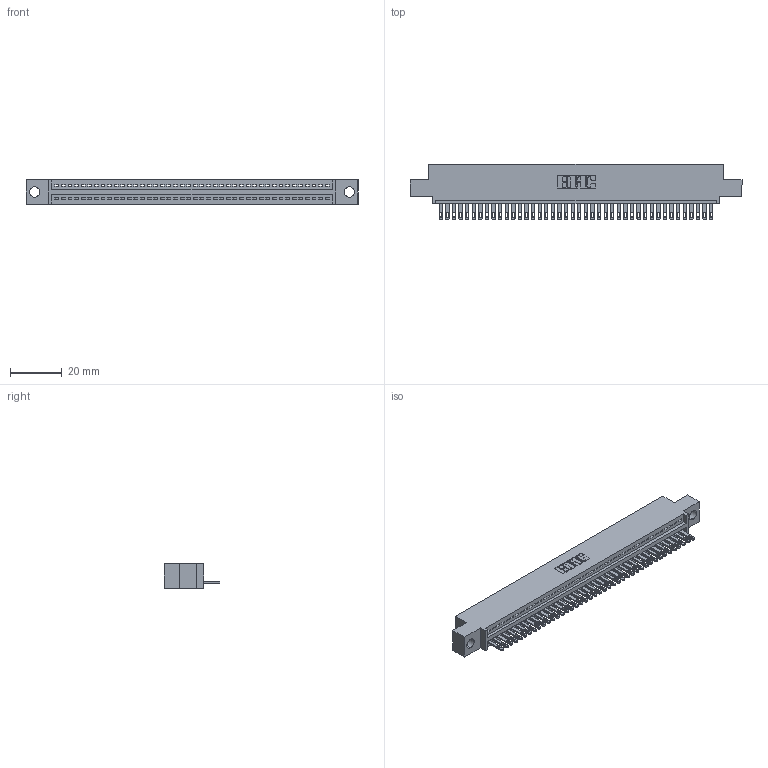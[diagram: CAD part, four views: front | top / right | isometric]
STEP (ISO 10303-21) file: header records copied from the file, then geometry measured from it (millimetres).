
FILE_DESCRIPTION (( 'STEP AP203' ), '1' );
FILE_NAME ('345-042-500-404.STEP', '2019-10-08T13:27:13', ( '' ), ( '' ), 'SwSTEP 2.0', 'SolidWorks 2016', '' );
FILE_SCHEMA (( 'CONFIG_CONTROL_DESIGN' ));
Length unit declared in the file: inch
Products named in the file (3): 345 Part_0.110 Offset - 0.156 Dia-TH; 345-042-500-404; 345-292-001_345-293-100
Assembly tree (43 placements, depth 2):
  345-042-500-404
    345 Part_0.110 Offset - 0.156 Dia-TH
    345-292-001_345-293-100  x42
Bounding box: 127.89 x 21.51 x 9.4 mm (x, y, z)
Volume: 12011.8 mm3; surface area: 15947.6 mm2
Topology: 43 solids, 43 shells, 2398 faces, 7409 edges, 4938 vertices
Faces by surface type: plane 1512, cylinder 886
Entity records: 31675 total; most frequent: CARTESIAN_POINT 5494, ORIENTED_EDGE 5470, DIRECTION 4799, EDGE_CURVE 2735, VECTOR 2431, LINE 2431, VERTEX_POINT 1822, AXIS2_PLACEMENT_3D 1184
